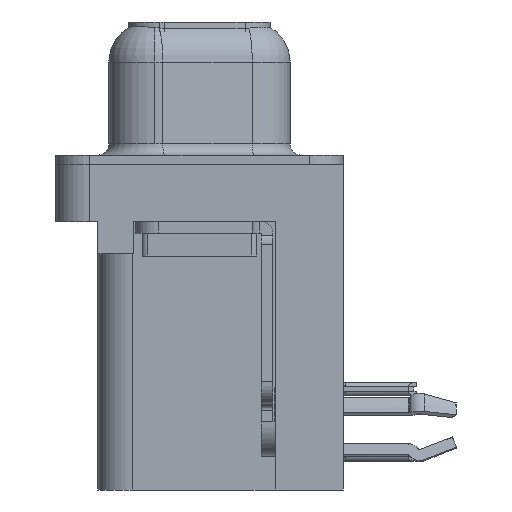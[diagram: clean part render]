
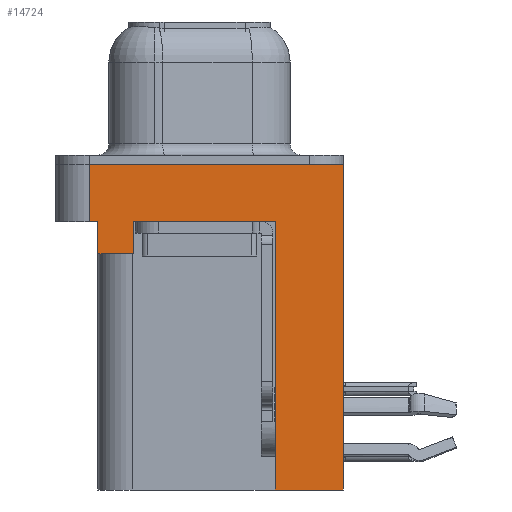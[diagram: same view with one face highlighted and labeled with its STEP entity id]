
A CAD part, left-side view. The second image highlights one B-rep face of the part: STEP entity #14724.
In plain terms, the highlighted planar face has unit normal (-1, 0, 0).
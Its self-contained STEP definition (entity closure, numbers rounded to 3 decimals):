
#568 = DIRECTION ( 'NONE',  ( 0., 1., 0. ) ) ;
#1024 = VECTOR ( 'NONE', #10652, 1000. ) ;
#1232 = ORIENTED_EDGE ( 'NONE', *, *, #29077, .F. ) ;
#2171 = LINE ( 'NONE', #25765, #9902 ) ;
#3323 = AXIS2_PLACEMENT_3D ( 'NONE', #14072, #18686, #6972 ) ;
#3537 = VECTOR ( 'NONE', #15111, 1000. ) ;
#3830 = CARTESIAN_POINT ( 'NONE',  ( -3., -6.275, -2.5 ) ) ;
#4323 = DIRECTION ( 'NONE',  ( 0., 0., 1. ) ) ;
#4364 = PLANE ( 'NONE',  #3323 ) ;
#5948 = VERTEX_POINT ( 'NONE', #6657 ) ;
#6007 = CARTESIAN_POINT ( 'NONE',  ( -3., 2.895, -3.9 ) ) ;
#6623 = ORIENTED_EDGE ( 'NONE', *, *, #21216, .F. ) ;
#6657 = CARTESIAN_POINT ( 'NONE',  ( -3., -6.275, -14.2 ) ) ;
#6668 = ORIENTED_EDGE ( 'NONE', *, *, #7973, .T. ) ;
#6972 = DIRECTION ( 'NONE',  ( 0., 0., 1. ) ) ;
#7051 = CARTESIAN_POINT ( 'NONE',  ( -3., 4.775, -2.5 ) ) ;
#7248 = LINE ( 'NONE', #16670, #29041 ) ;
#7349 = DIRECTION ( 'NONE',  ( 0., -1., 0. ) ) ;
#7400 = EDGE_CURVE ( 'NONE', #12329, #15345, #7248, .T. ) ;
#7632 = VERTEX_POINT ( 'NONE', #25004 ) ;
#7793 = LINE ( 'NONE', #16604, #11106 ) ;
#7973 = EDGE_CURVE ( 'NONE', #26429, #7632, #12918, .T. ) ;
#8162 = LINE ( 'NONE', #21737, #3537 ) ;
#8261 = VERTEX_POINT ( 'NONE', #12996 ) ;
#8960 = EDGE_CURVE ( 'NONE', #15345, #8261, #9808, .T. ) ;
#9370 = LINE ( 'NONE', #7051, #1024 ) ;
#9808 = LINE ( 'NONE', #18928, #19770 ) ;
#9844 = CARTESIAN_POINT ( 'NONE',  ( -3., 2.895, -2.5 ) ) ;
#9902 = VECTOR ( 'NONE', #4323, 1000. ) ;
#10247 = VERTEX_POINT ( 'NONE', #15828 ) ;
#10514 = DIRECTION ( 'NONE',  ( 0., 0., 1. ) ) ;
#10652 = DIRECTION ( 'NONE',  ( 0., 0., 1. ) ) ;
#11106 = VECTOR ( 'NONE', #568, 1000. ) ;
#11535 = ORIENTED_EDGE ( 'NONE', *, *, #18224, .F. ) ;
#12329 = VERTEX_POINT ( 'NONE', #6007 ) ;
#12734 = EDGE_CURVE ( 'NONE', #12329, #10247, #7793, .T. ) ;
#12918 = LINE ( 'NONE', #3830, #25094 ) ;
#12996 = CARTESIAN_POINT ( 'NONE',  ( -3., -3.295, -2.5 ) ) ;
#13327 = VECTOR ( 'NONE', #24716, 1000. ) ;
#13342 = EDGE_LOOP ( 'NONE', ( #11535, #20114, #6668, #28269, #23223, #20832, #19124, #6623, #1232, #22387 ) ) ;
#13359 = CARTESIAN_POINT ( 'NONE',  ( -3., -6.275, 0. ) ) ;
#13799 = DIRECTION ( 'NONE',  ( 0., -1., 0. ) ) ;
#14072 = CARTESIAN_POINT ( 'NONE',  ( -3., -6.275, -2.5 ) ) ;
#14724 = ADVANCED_FACE ( 'NONE', ( #27650 ), #4364, .T. ) ;
#15111 = DIRECTION ( 'NONE',  ( 0., 1., 0. ) ) ;
#15345 = VERTEX_POINT ( 'NONE', #9844 ) ;
#15828 = CARTESIAN_POINT ( 'NONE',  ( -3., 4.425, -3.9 ) ) ;
#16317 = CARTESIAN_POINT ( 'NONE',  ( -3., -3.295, -14.2 ) ) ;
#16604 = CARTESIAN_POINT ( 'NONE',  ( -3., 4.425, -3.9 ) ) ;
#16670 = CARTESIAN_POINT ( 'NONE',  ( -3., 2.895, -3.9 ) ) ;
#17445 = LINE ( 'NONE', #24564, #25183 ) ;
#17584 = LINE ( 'NONE', #22244, #13327 ) ;
#17977 = LINE ( 'NONE', #22626, #24101 ) ;
#18224 = EDGE_CURVE ( 'NONE', #27836, #28368, #17977, .T. ) ;
#18442 = CARTESIAN_POINT ( 'NONE',  ( -3., 4.775, -2.5 ) ) ;
#18686 = DIRECTION ( 'NONE',  ( -1., 0., 0. ) ) ;
#18928 = CARTESIAN_POINT ( 'NONE',  ( -3., -6.275, -2.5 ) ) ;
#19124 = ORIENTED_EDGE ( 'NONE', *, *, #8960, .T. ) ;
#19770 = VECTOR ( 'NONE', #7349, 1000. ) ;
#20114 = ORIENTED_EDGE ( 'NONE', *, *, #27959, .F. ) ;
#20832 = ORIENTED_EDGE ( 'NONE', *, *, #7400, .T. ) ;
#21216 = EDGE_CURVE ( 'NONE', #27929, #8261, #2171, .T. ) ;
#21737 = CARTESIAN_POINT ( 'NONE',  ( -3., -3.295, -14.2 ) ) ;
#21770 = CARTESIAN_POINT ( 'NONE',  ( -3., 4.775, 0. ) ) ;
#22244 = CARTESIAN_POINT ( 'NONE',  ( -3., -6.275, -2.5 ) ) ;
#22387 = ORIENTED_EDGE ( 'NONE', *, *, #27731, .T. ) ;
#22626 = CARTESIAN_POINT ( 'NONE',  ( -3., -6.275, 0. ) ) ;
#22790 = DIRECTION ( 'NONE',  ( 0., -1., 0. ) ) ;
#23223 = ORIENTED_EDGE ( 'NONE', *, *, #12734, .F. ) ;
#24101 = VECTOR ( 'NONE', #22790, 1000. ) ;
#24564 = CARTESIAN_POINT ( 'NONE',  ( -3., 4.425, -3.9 ) ) ;
#24716 = DIRECTION ( 'NONE',  ( 0., 0., 1. ) ) ;
#25004 = CARTESIAN_POINT ( 'NONE',  ( -3., 4.425, -2.5 ) ) ;
#25094 = VECTOR ( 'NONE', #13799, 1000. ) ;
#25183 = VECTOR ( 'NONE', #10514, 1000. ) ;
#25765 = CARTESIAN_POINT ( 'NONE',  ( -3., -3.295, -14.2 ) ) ;
#26429 = VERTEX_POINT ( 'NONE', #18442 ) ;
#26835 = DIRECTION ( 'NONE',  ( 0., 0., 1. ) ) ;
#27650 = FACE_OUTER_BOUND ( 'NONE', #13342, .T. ) ;
#27731 = EDGE_CURVE ( 'NONE', #5948, #28368, #17584, .T. ) ;
#27836 = VERTEX_POINT ( 'NONE', #21770 ) ;
#27929 = VERTEX_POINT ( 'NONE', #16317 ) ;
#27959 = EDGE_CURVE ( 'NONE', #26429, #27836, #9370, .T. ) ;
#28269 = ORIENTED_EDGE ( 'NONE', *, *, #29921, .F. ) ;
#28368 = VERTEX_POINT ( 'NONE', #13359 ) ;
#29041 = VECTOR ( 'NONE', #26835, 1000. ) ;
#29077 = EDGE_CURVE ( 'NONE', #5948, #27929, #8162, .T. ) ;
#29921 = EDGE_CURVE ( 'NONE', #10247, #7632, #17445, .T. ) ;
